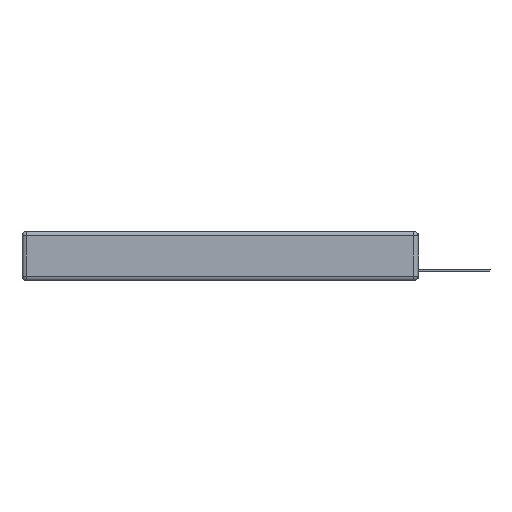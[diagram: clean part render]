
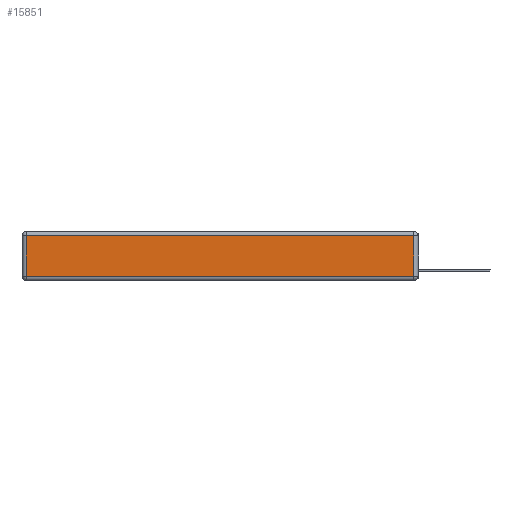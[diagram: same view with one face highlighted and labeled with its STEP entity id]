
A CAD part, left-side view. The second image highlights one B-rep face of the part: STEP entity #15851.
In plain terms, the highlighted planar face has unit normal (-1, 0, 0).
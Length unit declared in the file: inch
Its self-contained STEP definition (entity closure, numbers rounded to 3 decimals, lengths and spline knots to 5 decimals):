
#935 = LINE ( 'NONE', #7207, #13982 ) ;
#1358 = EDGE_CURVE ( 'NONE', #19339, #4237, #19687, .T. ) ;
#1824 = CARTESIAN_POINT ( 'NONE',  ( 0., 0., -0.343 ) ) ;
#3330 = DIRECTION ( 'NONE',  ( 0., 0., 1. ) ) ;
#3338 = ORIENTED_EDGE ( 'NONE', *, *, #16585, .T. ) ;
#3550 = LINE ( 'NONE', #11318, #9327 ) ;
#3580 = AXIS2_PLACEMENT_3D ( 'NONE', #1824, #17151, #3330 ) ;
#4118 = DIRECTION ( 'NONE',  ( 0., 0., 1. ) ) ;
#4146 = CARTESIAN_POINT ( 'NONE',  ( 0., 0.03, -0.03 ) ) ;
#4237 = VERTEX_POINT ( 'NONE', #19593 ) ;
#4572 = DIRECTION ( 'NONE',  ( 0., 0., -1. ) ) ;
#4878 = VECTOR ( 'NONE', #17923, 39.37008 ) ;
#4926 = EDGE_CURVE ( 'NONE', #4237, #8295, #3550, .T. ) ;
#6252 = CARTESIAN_POINT ( 'NONE',  ( 0., 2.72, -0.343 ) ) ;
#6401 = PLANE ( 'NONE',  #3580 ) ;
#6664 = LINE ( 'NONE', #14631, #4878 ) ;
#7034 = ORIENTED_EDGE ( 'NONE', *, *, #8404, .T. ) ;
#7207 = CARTESIAN_POINT ( 'NONE',  ( 0., 0.03, -0.343 ) ) ;
#8098 = VERTEX_POINT ( 'NONE', #4146 ) ;
#8295 = VERTEX_POINT ( 'NONE', #9616 ) ;
#8404 = EDGE_CURVE ( 'NONE', #8295, #8098, #935, .T. ) ;
#9309 = FACE_OUTER_BOUND ( 'NONE', #17494, .T. ) ;
#9327 = VECTOR ( 'NONE', #14790, 39.37008 ) ;
#9616 = CARTESIAN_POINT ( 'NONE',  ( 0., 0.03, -0.313 ) ) ;
#11318 = CARTESIAN_POINT ( 'NONE',  ( 0., 0., -0.313 ) ) ;
#13901 = ORIENTED_EDGE ( 'NONE', *, *, #4926, .T. ) ;
#13982 = VECTOR ( 'NONE', #4118, 39.37008 ) ;
#14631 = CARTESIAN_POINT ( 'NONE',  ( 0., 2.75, -0.03 ) ) ;
#14790 = DIRECTION ( 'NONE',  ( 0., -1., 0. ) ) ;
#15851 = ADVANCED_FACE ( 'NONE', ( #9309 ), #6401, .T. ) ;
#16463 = ORIENTED_EDGE ( 'NONE', *, *, #1358, .T. ) ;
#16585 = EDGE_CURVE ( 'NONE', #8098, #19339, #6664, .T. ) ;
#17151 = DIRECTION ( 'NONE',  ( -1., 0., 0. ) ) ;
#17494 = EDGE_LOOP ( 'NONE', ( #13901, #7034, #3338, #16463 ) ) ;
#17923 = DIRECTION ( 'NONE',  ( 0., 1., 0. ) ) ;
#18473 = CARTESIAN_POINT ( 'NONE',  ( 0., 2.72, -0.03 ) ) ;
#19339 = VERTEX_POINT ( 'NONE', #18473 ) ;
#19518 = VECTOR ( 'NONE', #4572, 39.37008 ) ;
#19593 = CARTESIAN_POINT ( 'NONE',  ( 0., 2.72, -0.313 ) ) ;
#19687 = LINE ( 'NONE', #6252, #19518 ) ;
